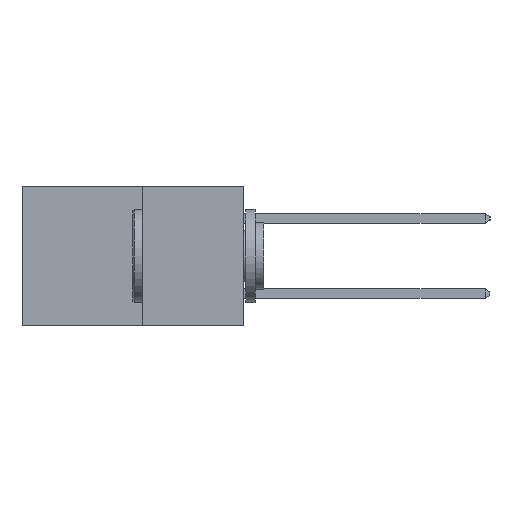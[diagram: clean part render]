
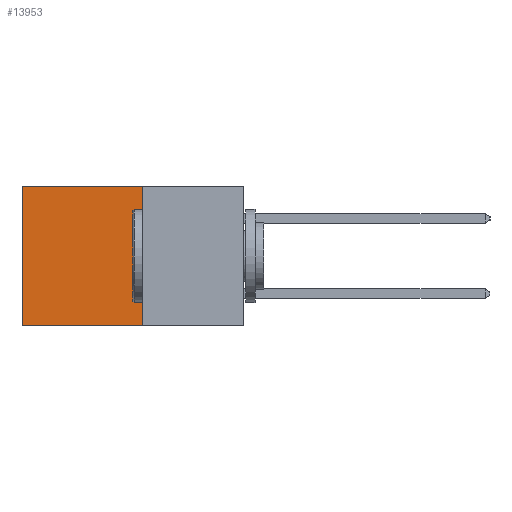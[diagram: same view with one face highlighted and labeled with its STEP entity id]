
A CAD part, left-side view. The second image highlights one B-rep face of the part: STEP entity #13953.
In plain terms, the highlighted planar face has unit normal (-1, 0, 0).
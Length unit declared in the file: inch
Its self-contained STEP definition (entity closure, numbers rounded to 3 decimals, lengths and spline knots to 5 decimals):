
#484 = CARTESIAN_POINT ( 'NONE',  ( 0.277, 0.59, -0.37 ) ) ;
#620 = CARTESIAN_POINT ( 'NONE',  ( 0.277, 0.27, 0. ) ) ;
#705 = FACE_OUTER_BOUND ( 'NONE', #15671, .T. ) ;
#852 = EDGE_CURVE ( 'NONE', #16354, #15366, #18363, .T. ) ;
#3109 = ORIENTED_EDGE ( 'NONE', *, *, #18315, .T. ) ;
#3489 = LINE ( 'NONE', #5706, #11973 ) ;
#4569 = CARTESIAN_POINT ( 'NONE',  ( 0.277, 0.27, -0.37 ) ) ;
#4595 = VECTOR ( 'NONE', #6397, 39.37008 ) ;
#4980 = VECTOR ( 'NONE', #21602, 39.37008 ) ;
#5038 = CARTESIAN_POINT ( 'NONE',  ( 0.277, 0.27, -0.37 ) ) ;
#5184 = LINE ( 'NONE', #620, #18050 ) ;
#5706 = CARTESIAN_POINT ( 'NONE',  ( 0.277, 0.27, -0.37 ) ) ;
#6311 = DIRECTION ( 'NONE',  ( 0., 0., -1. ) ) ;
#6397 = DIRECTION ( 'NONE',  ( 0., 0., -1. ) ) ;
#6440 = VERTEX_POINT ( 'NONE', #484 ) ;
#7737 = ORIENTED_EDGE ( 'NONE', *, *, #18821, .F. ) ;
#8248 = ORIENTED_EDGE ( 'NONE', *, *, #852, .F. ) ;
#8405 = CARTESIAN_POINT ( 'NONE',  ( 0.277, 0.59, 0. ) ) ;
#11973 = VECTOR ( 'NONE', #14041, 39.37008 ) ;
#12362 = EDGE_CURVE ( 'NONE', #16354, #13487, #5184, .T. ) ;
#12645 = ORIENTED_EDGE ( 'NONE', *, *, #12362, .T. ) ;
#12940 = AXIS2_PLACEMENT_3D ( 'NONE', #4569, #16309, #6311 ) ;
#13487 = VERTEX_POINT ( 'NONE', #8405 ) ;
#13953 = ADVANCED_FACE ( 'NONE', ( #705 ), #14614, .F. ) ;
#14041 = DIRECTION ( 'NONE',  ( 0., 1., 0. ) ) ;
#14614 = PLANE ( 'NONE',  #12940 ) ;
#14694 = CARTESIAN_POINT ( 'NONE',  ( 0.277, 0.59, -0.37 ) ) ;
#15366 = VERTEX_POINT ( 'NONE', #5038 ) ;
#15671 = EDGE_LOOP ( 'NONE', ( #3109, #7737, #8248, #12645 ) ) ;
#15871 = CARTESIAN_POINT ( 'NONE',  ( 0.277, 0.27, -0.37 ) ) ;
#16309 = DIRECTION ( 'NONE',  ( 1., 0., 0. ) ) ;
#16354 = VERTEX_POINT ( 'NONE', #19951 ) ;
#17488 = DIRECTION ( 'NONE',  ( 0., 1., 0. ) ) ;
#17976 = LINE ( 'NONE', #14694, #4595 ) ;
#18050 = VECTOR ( 'NONE', #17488, 39.37008 ) ;
#18315 = EDGE_CURVE ( 'NONE', #13487, #6440, #17976, .T. ) ;
#18363 = LINE ( 'NONE', #15871, #4980 ) ;
#18821 = EDGE_CURVE ( 'NONE', #15366, #6440, #3489, .T. ) ;
#19951 = CARTESIAN_POINT ( 'NONE',  ( 0.277, 0.27, 0. ) ) ;
#21602 = DIRECTION ( 'NONE',  ( 0., 0., -1. ) ) ;
